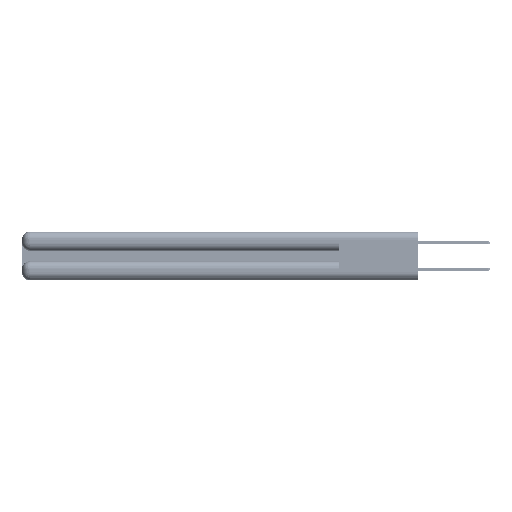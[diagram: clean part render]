
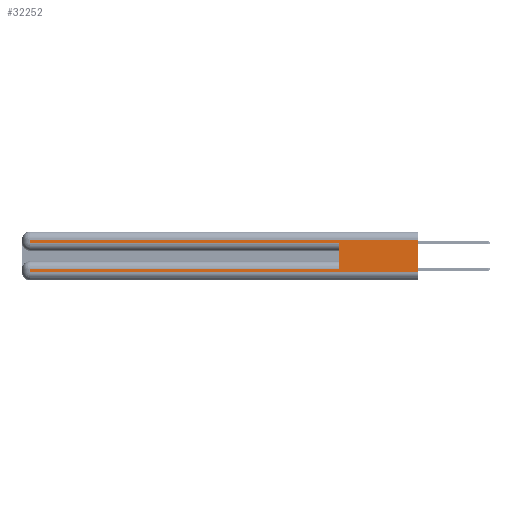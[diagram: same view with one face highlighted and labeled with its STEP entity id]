
A CAD part, left-side view. The second image highlights one B-rep face of the part: STEP entity #32252.
In plain terms, the highlighted planar face has unit normal (-1, 0, 0).
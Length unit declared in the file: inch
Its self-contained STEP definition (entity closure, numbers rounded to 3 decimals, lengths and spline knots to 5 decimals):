
#239 = EDGE_CURVE ( 'NONE', #53661, #27605, #42514, .T. ) ;
#240 = LINE ( 'NONE', #51925, #32400 ) ;
#2189 = CARTESIAN_POINT ( 'NONE',  ( 0., 2.94, 0.085 ) ) ;
#3503 = ORIENTED_EDGE ( 'NONE', *, *, #47184, .T. ) ;
#4177 = VECTOR ( 'NONE', #55617, 39.37008 ) ;
#4889 = LINE ( 'NONE', #42071, #26571 ) ;
#5279 = DIRECTION ( 'NONE',  ( 0., 1., 0. ) ) ;
#6126 = ORIENTED_EDGE ( 'NONE', *, *, #27636, .T. ) ;
#6750 = CARTESIAN_POINT ( 'NONE',  ( 0., 0., 0.06 ) ) ;
#6835 = FACE_OUTER_BOUND ( 'NONE', #45053, .T. ) ;
#7178 = PLANE ( 'NONE',  #36934 ) ;
#7351 = CARTESIAN_POINT ( 'NONE',  ( 0., 0.6, 0.145 ) ) ;
#9453 = ORIENTED_EDGE ( 'NONE', *, *, #46658, .T. ) ;
#11344 = DIRECTION ( 'NONE',  ( 0., -1., 0. ) ) ;
#11437 = LINE ( 'NONE', #7351, #28174 ) ;
#12222 = ORIENTED_EDGE ( 'NONE', *, *, #20108, .T. ) ;
#12482 = DIRECTION ( 'NONE',  ( 0., 0., -1. ) ) ;
#12527 = LINE ( 'NONE', #46091, #23664 ) ;
#16170 = DIRECTION ( 'NONE',  ( 0., 0., -1. ) ) ;
#17426 = ORIENTED_EDGE ( 'NONE', *, *, #34561, .T. ) ;
#20108 = EDGE_CURVE ( 'NONE', #40111, #43500, #240, .T. ) ;
#21025 = CARTESIAN_POINT ( 'NONE',  ( 0., 0.6, 0.285 ) ) ;
#21039 = DIRECTION ( 'NONE',  ( 0., 0., 1. ) ) ;
#21775 = CARTESIAN_POINT ( 'NONE',  ( 0., 2.94, 0.31 ) ) ;
#22123 = CARTESIAN_POINT ( 'NONE',  ( 0., 0., 0.31 ) ) ;
#23338 = ORIENTED_EDGE ( 'NONE', *, *, #239, .F. ) ;
#23664 = VECTOR ( 'NONE', #50720, 39.37008 ) ;
#24346 = CARTESIAN_POINT ( 'NONE',  ( 0., 0., 0.085 ) ) ;
#26125 = VECTOR ( 'NONE', #11344, 39.37008 ) ;
#26571 = VECTOR ( 'NONE', #43571, 39.37008 ) ;
#27605 = VERTEX_POINT ( 'NONE', #6750 ) ;
#27636 = EDGE_CURVE ( 'NONE', #32372, #40111, #44583, .T. ) ;
#28131 = ORIENTED_EDGE ( 'NONE', *, *, #51274, .F. ) ;
#28174 = VECTOR ( 'NONE', #21039, 39.37008 ) ;
#28898 = CARTESIAN_POINT ( 'NONE',  ( 0., 0., 0.06 ) ) ;
#29318 = VECTOR ( 'NONE', #35782, 39.37008 ) ;
#32252 = ADVANCED_FACE ( 'NONE', ( #6835 ), #7178, .F. ) ;
#32372 = VERTEX_POINT ( 'NONE', #39902 ) ;
#32400 = VECTOR ( 'NONE', #12482, 39.37008 ) ;
#34561 = EDGE_CURVE ( 'NONE', #43500, #27605, #51108, .T. ) ;
#34924 = CARTESIAN_POINT ( 'NONE',  ( 0., 2.94, 0.06 ) ) ;
#35782 = DIRECTION ( 'NONE',  ( 0., 0., -1. ) ) ;
#36934 = AXIS2_PLACEMENT_3D ( 'NONE', #46902, #38344, #16170 ) ;
#38344 = DIRECTION ( 'NONE',  ( 1., 0., 0. ) ) ;
#39706 = VERTEX_POINT ( 'NONE', #21775 ) ;
#39902 = CARTESIAN_POINT ( 'NONE',  ( 0., 0.6, 0.085 ) ) ;
#40111 = VERTEX_POINT ( 'NONE', #2189 ) ;
#40821 = CARTESIAN_POINT ( 'NONE',  ( 0., 0., 0.37 ) ) ;
#41469 = VECTOR ( 'NONE', #5279, 39.37008 ) ;
#42071 = CARTESIAN_POINT ( 'NONE',  ( 0., 0., 0.285 ) ) ;
#42514 = LINE ( 'NONE', #40821, #29318 ) ;
#42880 = VERTEX_POINT ( 'NONE', #21025 ) ;
#43500 = VERTEX_POINT ( 'NONE', #34924 ) ;
#43571 = DIRECTION ( 'NONE',  ( 0., -1., 0. ) ) ;
#44583 = LINE ( 'NONE', #24346, #4177 ) ;
#45053 = EDGE_LOOP ( 'NONE', ( #23338, #51475, #3503, #9453, #28131, #6126, #12222, #17426 ) ) ;
#46091 = CARTESIAN_POINT ( 'NONE',  ( 0., 2.94, 0.37 ) ) ;
#46658 = EDGE_CURVE ( 'NONE', #55766, #42880, #4889, .T. ) ;
#46902 = CARTESIAN_POINT ( 'NONE',  ( 0., 0., 0.37 ) ) ;
#47184 = EDGE_CURVE ( 'NONE', #39706, #55766, #12527, .T. ) ;
#49686 = CARTESIAN_POINT ( 'NONE',  ( 0., 2.94, 0.285 ) ) ;
#50375 = EDGE_CURVE ( 'NONE', #53661, #39706, #52587, .T. ) ;
#50607 = CARTESIAN_POINT ( 'NONE',  ( 0., 0., 0.31 ) ) ;
#50720 = DIRECTION ( 'NONE',  ( 0., 0., -1. ) ) ;
#51108 = LINE ( 'NONE', #28898, #26125 ) ;
#51274 = EDGE_CURVE ( 'NONE', #32372, #42880, #11437, .T. ) ;
#51475 = ORIENTED_EDGE ( 'NONE', *, *, #50375, .T. ) ;
#51925 = CARTESIAN_POINT ( 'NONE',  ( 0., 2.94, 0.37 ) ) ;
#52587 = LINE ( 'NONE', #50607, #41469 ) ;
#53661 = VERTEX_POINT ( 'NONE', #22123 ) ;
#55617 = DIRECTION ( 'NONE',  ( 0., 1., 0. ) ) ;
#55766 = VERTEX_POINT ( 'NONE', #49686 ) ;
